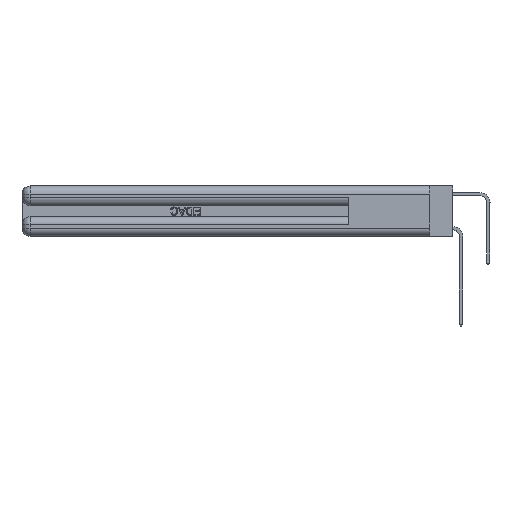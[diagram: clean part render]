
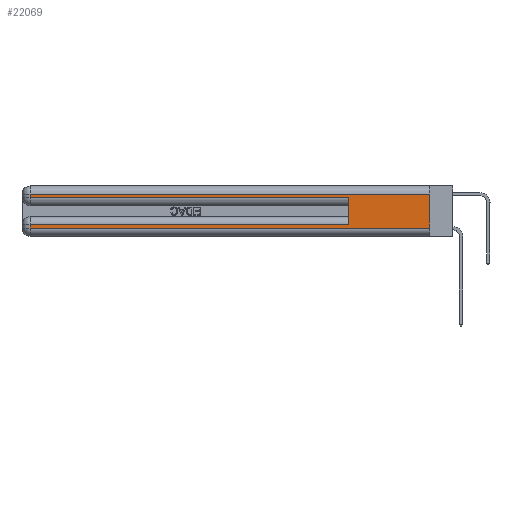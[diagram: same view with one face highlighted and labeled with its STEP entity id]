
A CAD part, left-side view. The second image highlights one B-rep face of the part: STEP entity #22069.
In plain terms, the highlighted planar face has unit normal (-1, 0, 0).
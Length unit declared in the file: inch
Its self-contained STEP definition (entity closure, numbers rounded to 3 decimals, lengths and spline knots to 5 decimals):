
#250 = DIRECTION ( 'NONE',  ( 0., 1., 0. ) ) ;
#710 = VECTOR ( 'NONE', #29476, 39.37008 ) ;
#822 = ORIENTED_EDGE ( 'NONE', *, *, #7533, .T. ) ;
#1678 = LINE ( 'NONE', #34559, #21592 ) ;
#1817 = VECTOR ( 'NONE', #14192, 39.37008 ) ;
#2847 = VECTOR ( 'NONE', #250, 39.37008 ) ;
#2853 = VERTEX_POINT ( 'NONE', #29633 ) ;
#3025 = LINE ( 'NONE', #34312, #7733 ) ;
#3494 = LINE ( 'NONE', #26040, #17031 ) ;
#3495 = CARTESIAN_POINT ( 'NONE',  ( 0., 2.94, 0.31 ) ) ;
#5578 = CARTESIAN_POINT ( 'NONE',  ( 0., 0., 0.06 ) ) ;
#5931 = ORIENTED_EDGE ( 'NONE', *, *, #30218, .T. ) ;
#6075 = LINE ( 'NONE', #30491, #1817 ) ;
#6667 = ORIENTED_EDGE ( 'NONE', *, *, #10515, .F. ) ;
#6954 = DIRECTION ( 'NONE',  ( 0., 1., 0. ) ) ;
#7533 = EDGE_CURVE ( 'NONE', #33160, #22555, #24559, .T. ) ;
#7733 = VECTOR ( 'NONE', #6954, 39.37008 ) ;
#7739 = CARTESIAN_POINT ( 'NONE',  ( 0., 0., 0.06 ) ) ;
#7911 = LINE ( 'NONE', #7739, #19287 ) ;
#9009 = CARTESIAN_POINT ( 'NONE',  ( 0., 0., 0.37 ) ) ;
#10515 = EDGE_CURVE ( 'NONE', #2853, #24319, #6075, .T. ) ;
#10634 = DIRECTION ( 'NONE',  ( 0., 0., 1. ) ) ;
#10920 = EDGE_CURVE ( 'NONE', #30768, #29111, #3494, .T. ) ;
#10982 = VERTEX_POINT ( 'NONE', #31399 ) ;
#11745 = AXIS2_PLACEMENT_3D ( 'NONE', #9009, #33762, #17032 ) ;
#12327 = EDGE_CURVE ( 'NONE', #29765, #10982, #1678, .T. ) ;
#13817 = LINE ( 'NONE', #24243, #710 ) ;
#14192 = DIRECTION ( 'NONE',  ( 0., 0., -1. ) ) ;
#14437 = CARTESIAN_POINT ( 'NONE',  ( 0., 0.6, 0.085 ) ) ;
#15497 = EDGE_CURVE ( 'NONE', #22555, #10982, #13817, .T. ) ;
#15671 = ORIENTED_EDGE ( 'NONE', *, *, #12327, .F. ) ;
#17031 = VECTOR ( 'NONE', #23787, 39.37008 ) ;
#17032 = DIRECTION ( 'NONE',  ( 0., 0., -1. ) ) ;
#18195 = VECTOR ( 'NONE', #18273, 39.37008 ) ;
#18273 = DIRECTION ( 'NONE',  ( 0., 0., -1. ) ) ;
#19287 = VECTOR ( 'NONE', #21287, 39.37008 ) ;
#19322 = LINE ( 'NONE', #22243, #2847 ) ;
#20338 = EDGE_LOOP ( 'NONE', ( #6667, #27412, #822, #23169, #15671, #34709, #25603, #5931 ) ) ;
#20537 = CARTESIAN_POINT ( 'NONE',  ( 0., 2.94, 0.085 ) ) ;
#21287 = DIRECTION ( 'NONE',  ( 0., -1., 0. ) ) ;
#21592 = VECTOR ( 'NONE', #10634, 39.37008 ) ;
#21968 = EDGE_CURVE ( 'NONE', #29765, #30768, #19322, .T. ) ;
#22069 = ADVANCED_FACE ( 'NONE', ( #29101 ), #30919, .F. ) ;
#22243 = CARTESIAN_POINT ( 'NONE',  ( 0., 0., 0.085 ) ) ;
#22555 = VERTEX_POINT ( 'NONE', #32689 ) ;
#23007 = CARTESIAN_POINT ( 'NONE',  ( 0., 2.94, 0.06 ) ) ;
#23169 = ORIENTED_EDGE ( 'NONE', *, *, #15497, .T. ) ;
#23787 = DIRECTION ( 'NONE',  ( 0., 0., -1. ) ) ;
#24243 = CARTESIAN_POINT ( 'NONE',  ( 0., 0., 0.285 ) ) ;
#24319 = VERTEX_POINT ( 'NONE', #5578 ) ;
#24559 = LINE ( 'NONE', #34425, #18195 ) ;
#25384 = EDGE_CURVE ( 'NONE', #2853, #33160, #3025, .T. ) ;
#25603 = ORIENTED_EDGE ( 'NONE', *, *, #10920, .T. ) ;
#26040 = CARTESIAN_POINT ( 'NONE',  ( 0., 2.94, 0.37 ) ) ;
#27412 = ORIENTED_EDGE ( 'NONE', *, *, #25384, .T. ) ;
#29101 = FACE_OUTER_BOUND ( 'NONE', #20338, .T. ) ;
#29111 = VERTEX_POINT ( 'NONE', #23007 ) ;
#29476 = DIRECTION ( 'NONE',  ( 0., -1., 0. ) ) ;
#29633 = CARTESIAN_POINT ( 'NONE',  ( 0., 0., 0.31 ) ) ;
#29765 = VERTEX_POINT ( 'NONE', #14437 ) ;
#30218 = EDGE_CURVE ( 'NONE', #29111, #24319, #7911, .T. ) ;
#30491 = CARTESIAN_POINT ( 'NONE',  ( 0., 0., 0.37 ) ) ;
#30768 = VERTEX_POINT ( 'NONE', #20537 ) ;
#30919 = PLANE ( 'NONE',  #11745 ) ;
#31399 = CARTESIAN_POINT ( 'NONE',  ( 0., 0.6, 0.285 ) ) ;
#32689 = CARTESIAN_POINT ( 'NONE',  ( 0., 2.94, 0.285 ) ) ;
#33160 = VERTEX_POINT ( 'NONE', #3495 ) ;
#33762 = DIRECTION ( 'NONE',  ( 1., 0., 0. ) ) ;
#34312 = CARTESIAN_POINT ( 'NONE',  ( 0., 0., 0.31 ) ) ;
#34425 = CARTESIAN_POINT ( 'NONE',  ( 0., 2.94, 0.37 ) ) ;
#34559 = CARTESIAN_POINT ( 'NONE',  ( 0., 0.6, 0.145 ) ) ;
#34709 = ORIENTED_EDGE ( 'NONE', *, *, #21968, .T. ) ;
